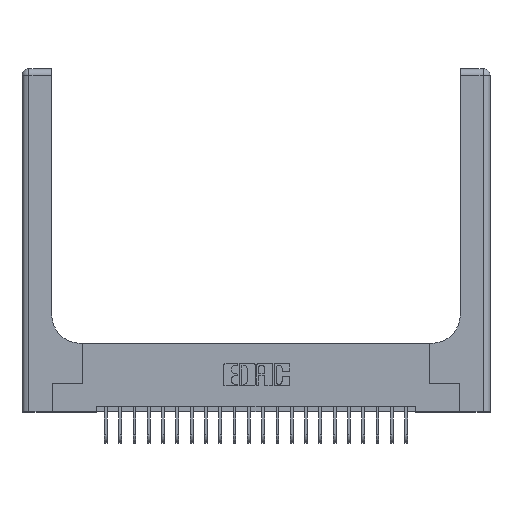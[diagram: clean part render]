
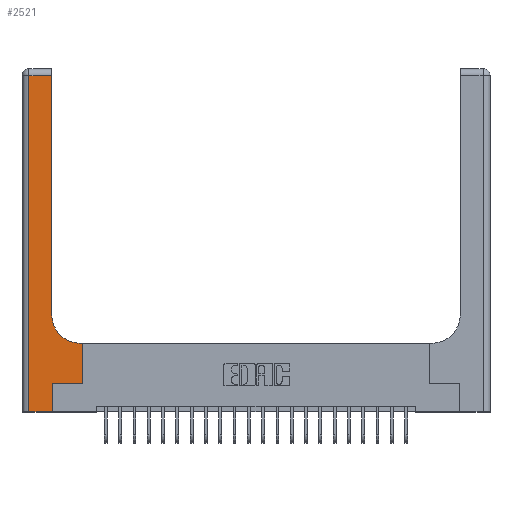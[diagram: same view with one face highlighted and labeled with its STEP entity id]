
A CAD part, top view. The second image highlights one B-rep face of the part: STEP entity #2521.
In plain terms, the highlighted planar face has unit normal (0, 0, 1).
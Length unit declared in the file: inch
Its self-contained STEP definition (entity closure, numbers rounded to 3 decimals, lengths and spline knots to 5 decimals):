
#12 = EDGE_LOOP ( 'NONE', ( #4691, #17816, #8330, #2130, #8799, #3658, #20602, #21157, #2725 ) ) ;
#142 = EDGE_CURVE ( 'NONE', #8635, #12308, #16857, .T. ) ;
#339 = DIRECTION ( 'NONE',  ( 0., 1., 0. ) ) ;
#989 = EDGE_CURVE ( 'NONE', #9791, #21868, #12962, .T. ) ;
#1738 = EDGE_CURVE ( 'NONE', #20033, #9791, #19430, .T. ) ;
#1918 = EDGE_CURVE ( 'NONE', #8031, #8635, #13463, .T. ) ;
#2130 = ORIENTED_EDGE ( 'NONE', *, *, #989, .T. ) ;
#2187 = DIRECTION ( 'NONE',  ( 0., 0., -1. ) ) ;
#2323 = LINE ( 'NONE', #7221, #5608 ) ;
#2354 = VECTOR ( 'NONE', #7587, 39.37008 ) ;
#2493 = CARTESIAN_POINT ( 'NONE',  ( 0.51, 0.6, 0.37 ) ) ;
#2521 = ADVANCED_FACE ( 'NONE', ( #19016 ), #12071, .F. ) ;
#2725 = ORIENTED_EDGE ( 'NONE', *, *, #6163, .T. ) ;
#3055 = CARTESIAN_POINT ( 'NONE',  ( 0.528, 0.25, 0.37 ) ) ;
#3323 = VERTEX_POINT ( 'NONE', #18403 ) ;
#3338 = VERTEX_POINT ( 'NONE', #20329 ) ;
#3658 = ORIENTED_EDGE ( 'NONE', *, *, #1918, .T. ) ;
#3727 = CARTESIAN_POINT ( 'NONE',  ( 0., 2.94, 0.37 ) ) ;
#3751 = CARTESIAN_POINT ( 'NONE',  ( 0.265, 0., 0.37 ) ) ;
#4145 = CARTESIAN_POINT ( 'NONE',  ( 0.06, 3., 0.37 ) ) ;
#4691 = ORIENTED_EDGE ( 'NONE', *, *, #12575, .T. ) ;
#4906 = CARTESIAN_POINT ( 'NONE',  ( 0.265, 0., 0.37 ) ) ;
#5504 = CARTESIAN_POINT ( 'NONE',  ( 0., 3., 0.37 ) ) ;
#5608 = VECTOR ( 'NONE', #339, 39.37008 ) ;
#5632 = LINE ( 'NONE', #3751, #9526 ) ;
#6163 = EDGE_CURVE ( 'NONE', #14366, #3323, #21371, .T. ) ;
#6348 = CARTESIAN_POINT ( 'NONE',  ( 0.265, 0.25, 0.37 ) ) ;
#6610 = DIRECTION ( 'NONE',  ( 0., 1., 0. ) ) ;
#7221 = CARTESIAN_POINT ( 'NONE',  ( 0.26, 3., 0.37 ) ) ;
#7504 = LINE ( 'NONE', #3727, #16622 ) ;
#7534 = CARTESIAN_POINT ( 'NONE',  ( 0., 0., 0.37 ) ) ;
#7582 = EDGE_CURVE ( 'NONE', #12308, #14366, #20961, .T. ) ;
#7587 = DIRECTION ( 'NONE',  ( 0., -1., 0. ) ) ;
#8031 = VERTEX_POINT ( 'NONE', #17440 ) ;
#8330 = ORIENTED_EDGE ( 'NONE', *, *, #1738, .T. ) ;
#8635 = VERTEX_POINT ( 'NONE', #20218 ) ;
#8799 = ORIENTED_EDGE ( 'NONE', *, *, #10461, .T. ) ;
#8927 = CARTESIAN_POINT ( 'NONE',  ( 0.528, 0.6, 0.37 ) ) ;
#9375 = CARTESIAN_POINT ( 'NONE',  ( 0.06, 0., 0.37 ) ) ;
#9526 = VECTOR ( 'NONE', #12529, 39.37008 ) ;
#9791 = VERTEX_POINT ( 'NONE', #9375 ) ;
#10461 = EDGE_CURVE ( 'NONE', #21868, #8031, #5632, .T. ) ;
#10630 = AXIS2_PLACEMENT_3D ( 'NONE', #10759, #19278, #10976 ) ;
#10759 = CARTESIAN_POINT ( 'NONE',  ( 0.51, 0.85, 0.37 ) ) ;
#10976 = DIRECTION ( 'NONE',  ( 1., 0., 0. ) ) ;
#11018 = VECTOR ( 'NONE', #6610, 39.37008 ) ;
#11669 = AXIS2_PLACEMENT_3D ( 'NONE', #5504, #2187, #12406 ) ;
#11966 = EDGE_CURVE ( 'NONE', #3338, #20033, #7504, .T. ) ;
#12071 = PLANE ( 'NONE',  #11669 ) ;
#12308 = VERTEX_POINT ( 'NONE', #8927 ) ;
#12406 = DIRECTION ( 'NONE',  ( -1., 0., 0. ) ) ;
#12529 = DIRECTION ( 'NONE',  ( 0., 1., 0. ) ) ;
#12575 = EDGE_CURVE ( 'NONE', #3323, #3338, #2323, .T. ) ;
#12959 = VECTOR ( 'NONE', #20852, 39.37008 ) ;
#12962 = LINE ( 'NONE', #7534, #16084 ) ;
#13130 = DIRECTION ( 'NONE',  ( 1., 0., 0. ) ) ;
#13463 = LINE ( 'NONE', #6348, #15489 ) ;
#13635 = CARTESIAN_POINT ( 'NONE',  ( 0.06, 2.94, 0.37 ) ) ;
#14366 = VERTEX_POINT ( 'NONE', #2493 ) ;
#15489 = VECTOR ( 'NONE', #13130, 39.37008 ) ;
#16084 = VECTOR ( 'NONE', #18126, 39.37008 ) ;
#16622 = VECTOR ( 'NONE', #17427, 39.37008 ) ;
#16857 = LINE ( 'NONE', #3055, #11018 ) ;
#17427 = DIRECTION ( 'NONE',  ( -1., 0., 0. ) ) ;
#17440 = CARTESIAN_POINT ( 'NONE',  ( 0.265, 0.25, 0.37 ) ) ;
#17465 = CARTESIAN_POINT ( 'NONE',  ( 0.26, 0.6, 0.37 ) ) ;
#17816 = ORIENTED_EDGE ( 'NONE', *, *, #11966, .T. ) ;
#18126 = DIRECTION ( 'NONE',  ( 1., 0., 0. ) ) ;
#18403 = CARTESIAN_POINT ( 'NONE',  ( 0.26, 0.85, 0.37 ) ) ;
#19016 = FACE_OUTER_BOUND ( 'NONE', #12, .T. ) ;
#19278 = DIRECTION ( 'NONE',  ( 0., 0., -1. ) ) ;
#19430 = LINE ( 'NONE', #4145, #2354 ) ;
#20033 = VERTEX_POINT ( 'NONE', #13635 ) ;
#20218 = CARTESIAN_POINT ( 'NONE',  ( 0.528, 0.25, 0.37 ) ) ;
#20329 = CARTESIAN_POINT ( 'NONE',  ( 0.26, 2.94, 0.37 ) ) ;
#20602 = ORIENTED_EDGE ( 'NONE', *, *, #142, .T. ) ;
#20852 = DIRECTION ( 'NONE',  ( -1., 0., 0. ) ) ;
#20961 = LINE ( 'NONE', #17465, #12959 ) ;
#21157 = ORIENTED_EDGE ( 'NONE', *, *, #7582, .T. ) ;
#21371 = CIRCLE ( 'NONE', #10630, 0.25 ) ;
#21868 = VERTEX_POINT ( 'NONE', #4906 ) ;
